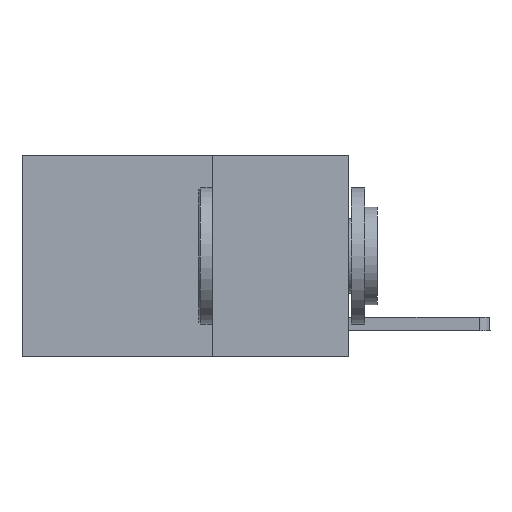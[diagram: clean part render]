
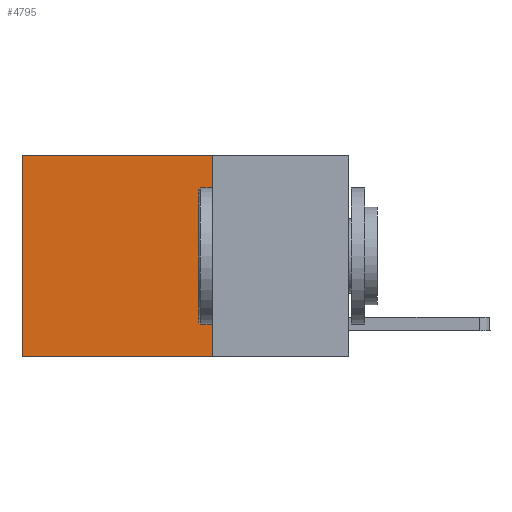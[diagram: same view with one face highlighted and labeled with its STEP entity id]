
A CAD part, left-side view. The second image highlights one B-rep face of the part: STEP entity #4795.
In plain terms, the highlighted planar face has unit normal (-1, 0, 0).
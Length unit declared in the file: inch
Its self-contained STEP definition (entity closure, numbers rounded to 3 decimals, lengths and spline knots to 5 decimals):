
#572 = EDGE_LOOP ( 'NONE', ( #9671, #2884, #2981, #2241 ) ) ;
#950 = CARTESIAN_POINT ( 'NONE',  ( 0.2625, 0.25, -0.37 ) ) ;
#989 = VECTOR ( 'NONE', #2173, 39.37008 ) ;
#1214 = CARTESIAN_POINT ( 'NONE',  ( 0.2625, 0.25, 0. ) ) ;
#1255 = AXIS2_PLACEMENT_3D ( 'NONE', #1214, #1269, #7426 ) ;
#1269 = DIRECTION ( 'NONE',  ( 1., 0., 0. ) ) ;
#1502 = VERTEX_POINT ( 'NONE', #4537 ) ;
#1700 = EDGE_CURVE ( 'NONE', #7912, #8864, #6418, .T. ) ;
#2002 = VERTEX_POINT ( 'NONE', #2463 ) ;
#2173 = DIRECTION ( 'NONE',  ( 0., 0., -1. ) ) ;
#2241 = ORIENTED_EDGE ( 'NONE', *, *, #2530, .T. ) ;
#2463 = CARTESIAN_POINT ( 'NONE',  ( 0.2625, 0.6, 0. ) ) ;
#2530 = EDGE_CURVE ( 'NONE', #1502, #2002, #6626, .T. ) ;
#2884 = ORIENTED_EDGE ( 'NONE', *, *, #1700, .F. ) ;
#2981 = ORIENTED_EDGE ( 'NONE', *, *, #5719, .F. ) ;
#4224 = CARTESIAN_POINT ( 'NONE',  ( 0.2625, 0.25, -0.37 ) ) ;
#4537 = CARTESIAN_POINT ( 'NONE',  ( 0.2625, 0.25, 0. ) ) ;
#4795 = ADVANCED_FACE ( 'NONE', ( #8076 ), #8179, .F. ) ;
#5198 = CARTESIAN_POINT ( 'NONE',  ( 0.2625, 0.25, 0. ) ) ;
#5719 = EDGE_CURVE ( 'NONE', #1502, #7912, #7101, .T. ) ;
#5805 = DIRECTION ( 'NONE',  ( 0., 1., 0. ) ) ;
#6018 = CARTESIAN_POINT ( 'NONE',  ( 0.2625, 0.6, 0. ) ) ;
#6352 = DIRECTION ( 'NONE',  ( 0., 0., -1. ) ) ;
#6418 = LINE ( 'NONE', #950, #9444 ) ;
#6626 = LINE ( 'NONE', #5198, #9764 ) ;
#7001 = EDGE_CURVE ( 'NONE', #2002, #8864, #9060, .T. ) ;
#7101 = LINE ( 'NONE', #9274, #8186 ) ;
#7426 = DIRECTION ( 'NONE',  ( 0., 0., -1. ) ) ;
#7912 = VERTEX_POINT ( 'NONE', #4224 ) ;
#8076 = FACE_OUTER_BOUND ( 'NONE', #572, .T. ) ;
#8179 = PLANE ( 'NONE',  #1255 ) ;
#8186 = VECTOR ( 'NONE', #6352, 39.37008 ) ;
#8602 = DIRECTION ( 'NONE',  ( 0., 1., 0. ) ) ;
#8864 = VERTEX_POINT ( 'NONE', #8934 ) ;
#8934 = CARTESIAN_POINT ( 'NONE',  ( 0.2625, 0.6, -0.37 ) ) ;
#9060 = LINE ( 'NONE', #6018, #989 ) ;
#9274 = CARTESIAN_POINT ( 'NONE',  ( 0.2625, 0.25, 0. ) ) ;
#9444 = VECTOR ( 'NONE', #8602, 39.37008 ) ;
#9671 = ORIENTED_EDGE ( 'NONE', *, *, #7001, .T. ) ;
#9764 = VECTOR ( 'NONE', #5805, 39.37008 ) ;
